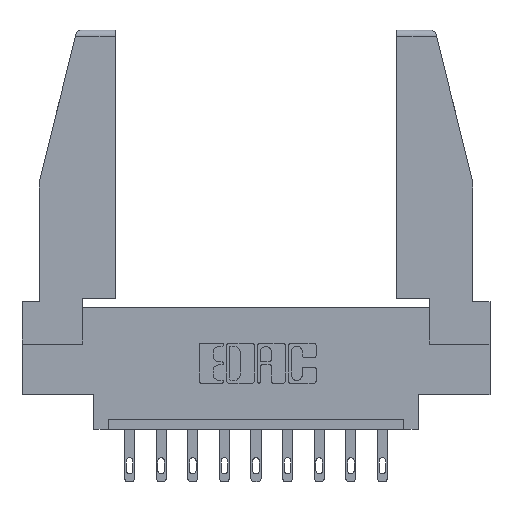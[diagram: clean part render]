
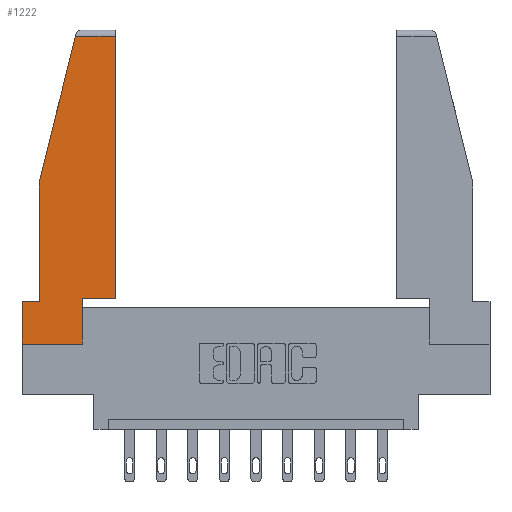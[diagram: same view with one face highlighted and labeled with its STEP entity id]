
A CAD part, top view. The second image highlights one B-rep face of the part: STEP entity #1222.
In plain terms, the highlighted planar face has unit normal (0, 0, 1).
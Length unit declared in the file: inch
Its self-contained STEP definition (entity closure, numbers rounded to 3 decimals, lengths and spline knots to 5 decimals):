
#244 = DIRECTION ( 'NONE',  ( 0., -1., 0. ) ) ;
#895 = VECTOR ( 'NONE', #7240, 39.37008 ) ;
#905 = CARTESIAN_POINT ( 'NONE',  ( 0.461, 0.223, 0. ) ) ;
#1032 = DIRECTION ( 'NONE',  ( 1., 0., 0. ) ) ;
#1222 = ADVANCED_FACE ( 'NONE', ( #7772 ), #2895, .T. ) ;
#1230 = ORIENTED_EDGE ( 'NONE', *, *, #12545, .T. ) ;
#1373 = CARTESIAN_POINT ( 'NONE',  ( 0.461, 1.52, 0. ) ) ;
#1715 = LINE ( 'NONE', #11696, #2684 ) ;
#1833 = EDGE_CURVE ( 'NONE', #13476, #8863, #11829, .T. ) ;
#1849 = LINE ( 'NONE', #9994, #5268 ) ;
#1947 = DIRECTION ( 'NONE',  ( 0., 1., 0. ) ) ;
#2038 = CARTESIAN_POINT ( 'NONE',  ( 0.2636, 1.52, 0. ) ) ;
#2073 = VERTEX_POINT ( 'NONE', #8009 ) ;
#2087 = VERTEX_POINT ( 'NONE', #12726 ) ;
#2328 = EDGE_CURVE ( 'NONE', #9030, #7703, #10518, .T. ) ;
#2439 = DIRECTION ( 'NONE',  ( -1., 0., 0. ) ) ;
#2476 = VECTOR ( 'NONE', #2439, 39.37008 ) ;
#2684 = VECTOR ( 'NONE', #8400, 39.37008 ) ;
#2895 = PLANE ( 'NONE',  #5851 ) ;
#3660 = CARTESIAN_POINT ( 'NONE',  ( 0., 0.21, 0. ) ) ;
#3678 = EDGE_CURVE ( 'NONE', #13219, #2087, #5102, .T. ) ;
#3709 = EDGE_CURVE ( 'NONE', #8863, #2073, #9655, .T. ) ;
#4611 = VERTEX_POINT ( 'NONE', #6751 ) ;
#4732 = ORIENTED_EDGE ( 'NONE', *, *, #12457, .T. ) ;
#5102 = LINE ( 'NONE', #7445, #2476 ) ;
#5268 = VECTOR ( 'NONE', #5657, 39.37008 ) ;
#5378 = DIRECTION ( 'NONE',  ( -0.239, -0.971, 0. ) ) ;
#5590 = VECTOR ( 'NONE', #5378, 39.37008 ) ;
#5657 = DIRECTION ( 'NONE',  ( 1., 0., 0. ) ) ;
#5677 = CARTESIAN_POINT ( 'NONE',  ( 0.297, 0.223, 0. ) ) ;
#5851 = AXIS2_PLACEMENT_3D ( 'NONE', #11476, #6287, #1032 ) ;
#6287 = DIRECTION ( 'NONE',  ( 0., 0., 1. ) ) ;
#6565 = ORIENTED_EDGE ( 'NONE', *, *, #2328, .T. ) ;
#6751 = CARTESIAN_POINT ( 'NONE',  ( 0., 0., 0. ) ) ;
#6936 = EDGE_CURVE ( 'NONE', #7864, #13476, #7542, .T. ) ;
#7240 = DIRECTION ( 'NONE',  ( 0., 1., 0. ) ) ;
#7420 = DIRECTION ( 'NONE',  ( -1., 0., 0. ) ) ;
#7445 = CARTESIAN_POINT ( 'NONE',  ( 0., 0.21, 0. ) ) ;
#7542 = LINE ( 'NONE', #905, #895 ) ;
#7549 = LINE ( 'NONE', #12568, #13101 ) ;
#7618 = CARTESIAN_POINT ( 'NONE',  ( 0.297, 0., 0. ) ) ;
#7703 = VERTEX_POINT ( 'NONE', #5677 ) ;
#7772 = FACE_OUTER_BOUND ( 'NONE', #11093, .T. ) ;
#7864 = VERTEX_POINT ( 'NONE', #12004 ) ;
#8009 = CARTESIAN_POINT ( 'NONE',  ( 0.086, 0.8, 0. ) ) ;
#8400 = DIRECTION ( 'NONE',  ( 1., 0., 0. ) ) ;
#8863 = VERTEX_POINT ( 'NONE', #2038 ) ;
#9030 = VERTEX_POINT ( 'NONE', #7618 ) ;
#9375 = CARTESIAN_POINT ( 'NONE',  ( 0., 1.52, 0. ) ) ;
#9655 = LINE ( 'NONE', #9750, #5590 ) ;
#9750 = CARTESIAN_POINT ( 'NONE',  ( 0.271, 1.55, 0. ) ) ;
#9971 = ORIENTED_EDGE ( 'NONE', *, *, #11119, .T. ) ;
#9994 = CARTESIAN_POINT ( 'NONE',  ( 0.297, 0.223, 0. ) ) ;
#10518 = LINE ( 'NONE', #12450, #13437 ) ;
#10763 = LINE ( 'NONE', #3660, #13249 ) ;
#10932 = ORIENTED_EDGE ( 'NONE', *, *, #6936, .T. ) ;
#11093 = EDGE_LOOP ( 'NONE', ( #10932, #11649, #13116, #4732, #12942, #9971, #1230, #6565, #13487 ) ) ;
#11119 = EDGE_CURVE ( 'NONE', #2087, #4611, #10763, .T. ) ;
#11476 = CARTESIAN_POINT ( 'NONE',  ( 0., 0., 0. ) ) ;
#11649 = ORIENTED_EDGE ( 'NONE', *, *, #1833, .T. ) ;
#11696 = CARTESIAN_POINT ( 'NONE',  ( 0., 0., 0. ) ) ;
#11829 = LINE ( 'NONE', #9375, #13456 ) ;
#12004 = CARTESIAN_POINT ( 'NONE',  ( 0.461, 0.223, 0. ) ) ;
#12450 = CARTESIAN_POINT ( 'NONE',  ( 0.297, 0., 0. ) ) ;
#12457 = EDGE_CURVE ( 'NONE', #2073, #13219, #7549, .T. ) ;
#12545 = EDGE_CURVE ( 'NONE', #4611, #9030, #1715, .T. ) ;
#12568 = CARTESIAN_POINT ( 'NONE',  ( 0.086, 0.8, 0. ) ) ;
#12726 = CARTESIAN_POINT ( 'NONE',  ( 0., 0.21, 0. ) ) ;
#12942 = ORIENTED_EDGE ( 'NONE', *, *, #3678, .T. ) ;
#12984 = DIRECTION ( 'NONE',  ( 0., -1., 0. ) ) ;
#13101 = VECTOR ( 'NONE', #244, 39.37008 ) ;
#13116 = ORIENTED_EDGE ( 'NONE', *, *, #3709, .T. ) ;
#13219 = VERTEX_POINT ( 'NONE', #13439 ) ;
#13249 = VECTOR ( 'NONE', #12984, 39.37008 ) ;
#13343 = EDGE_CURVE ( 'NONE', #7703, #7864, #1849, .T. ) ;
#13437 = VECTOR ( 'NONE', #1947, 39.37008 ) ;
#13439 = CARTESIAN_POINT ( 'NONE',  ( 0.086, 0.21, 0. ) ) ;
#13456 = VECTOR ( 'NONE', #7420, 39.37008 ) ;
#13476 = VERTEX_POINT ( 'NONE', #1373 ) ;
#13487 = ORIENTED_EDGE ( 'NONE', *, *, #13343, .T. ) ;
